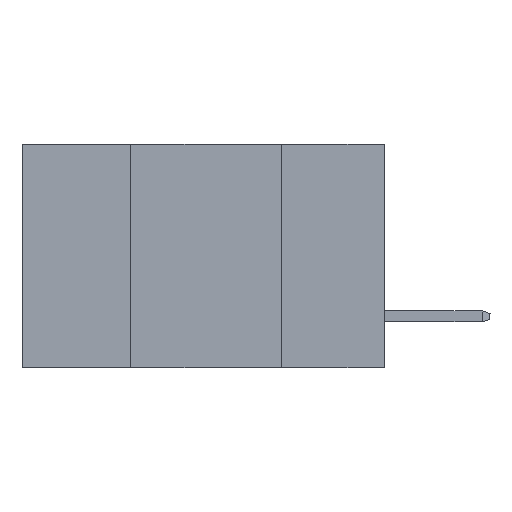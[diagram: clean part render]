
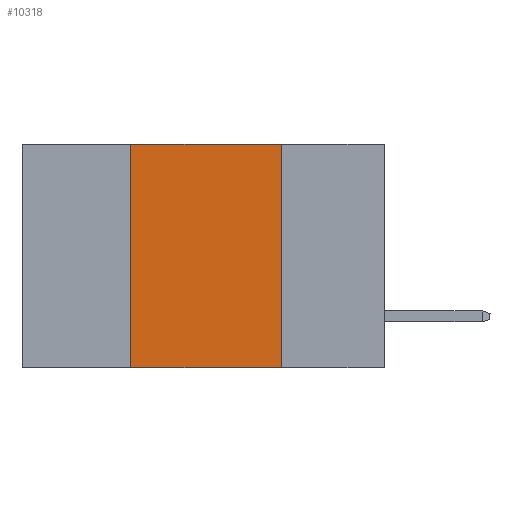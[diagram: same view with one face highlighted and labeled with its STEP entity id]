
A CAD part, left-side view. The second image highlights one B-rep face of the part: STEP entity #10318.
In plain terms, the highlighted planar face has unit normal (-1, 0, 0).
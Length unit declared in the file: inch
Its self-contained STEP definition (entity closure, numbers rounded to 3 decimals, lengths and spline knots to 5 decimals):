
#293 = EDGE_CURVE ( 'NONE', #9473, #713, #2386, .T. ) ;
#575 = ORIENTED_EDGE ( 'NONE', *, *, #6922, .F. ) ;
#713 = VERTEX_POINT ( 'NONE', #9090 ) ;
#1378 = PLANE ( 'NONE',  #9182 ) ;
#1427 = CARTESIAN_POINT ( 'NONE',  ( 0., 0.17, 0. ) ) ;
#1923 = CARTESIAN_POINT ( 'NONE',  ( 0., 0.6, 0. ) ) ;
#1928 = ORIENTED_EDGE ( 'NONE', *, *, #293, .T. ) ;
#2107 = VECTOR ( 'NONE', #10006, 39.37008 ) ;
#2381 = DIRECTION ( 'NONE',  ( 0., 0., -1. ) ) ;
#2386 = LINE ( 'NONE', #2831, #2107 ) ;
#2711 = LINE ( 'NONE', #9344, #7303 ) ;
#2831 = CARTESIAN_POINT ( 'NONE',  ( 0., 0.6, -0.37 ) ) ;
#3756 = FACE_OUTER_BOUND ( 'NONE', #8034, .T. ) ;
#3771 = ORIENTED_EDGE ( 'NONE', *, *, #10619, .F. ) ;
#3986 = VERTEX_POINT ( 'NONE', #1427 ) ;
#4698 = VECTOR ( 'NONE', #6433, 39.37008 ) ;
#5038 = DIRECTION ( 'NONE',  ( 1., 0., 0. ) ) ;
#5808 = CARTESIAN_POINT ( 'NONE',  ( 0., 0.42, -0.37 ) ) ;
#6433 = DIRECTION ( 'NONE',  ( 0., 0., -1. ) ) ;
#6858 = EDGE_CURVE ( 'NONE', #3986, #713, #10634, .T. ) ;
#6922 = EDGE_CURVE ( 'NONE', #9874, #3986, #11602, .T. ) ;
#7303 = VECTOR ( 'NONE', #7567, 39.37008 ) ;
#7567 = DIRECTION ( 'NONE',  ( 0., 0., 1. ) ) ;
#8034 = EDGE_LOOP ( 'NONE', ( #9371, #575, #3771, #1928 ) ) ;
#8524 = CARTESIAN_POINT ( 'NONE',  ( 0., 0.42, 0. ) ) ;
#8692 = CARTESIAN_POINT ( 'NONE',  ( 0., 0.6, 0. ) ) ;
#9035 = DIRECTION ( 'NONE',  ( 0., -1., 0. ) ) ;
#9090 = CARTESIAN_POINT ( 'NONE',  ( 0., 0.17, -0.37 ) ) ;
#9138 = CARTESIAN_POINT ( 'NONE',  ( 0., 0.17, 0. ) ) ;
#9182 = AXIS2_PLACEMENT_3D ( 'NONE', #8692, #5038, #2381 ) ;
#9344 = CARTESIAN_POINT ( 'NONE',  ( 0., 0.42, 0. ) ) ;
#9371 = ORIENTED_EDGE ( 'NONE', *, *, #6858, .F. ) ;
#9473 = VERTEX_POINT ( 'NONE', #5808 ) ;
#9874 = VERTEX_POINT ( 'NONE', #8524 ) ;
#10006 = DIRECTION ( 'NONE',  ( 0., -1., 0. ) ) ;
#10318 = ADVANCED_FACE ( 'NONE', ( #3756 ), #1378, .F. ) ;
#10619 = EDGE_CURVE ( 'NONE', #9473, #9874, #2711, .T. ) ;
#10634 = LINE ( 'NONE', #9138, #4698 ) ;
#11340 = VECTOR ( 'NONE', #9035, 39.37008 ) ;
#11602 = LINE ( 'NONE', #1923, #11340 ) ;
